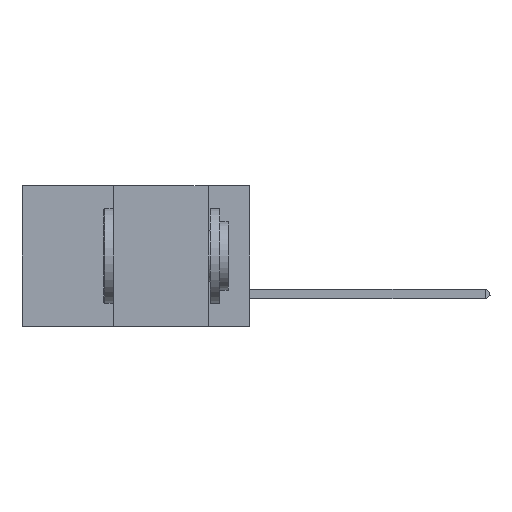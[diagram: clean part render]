
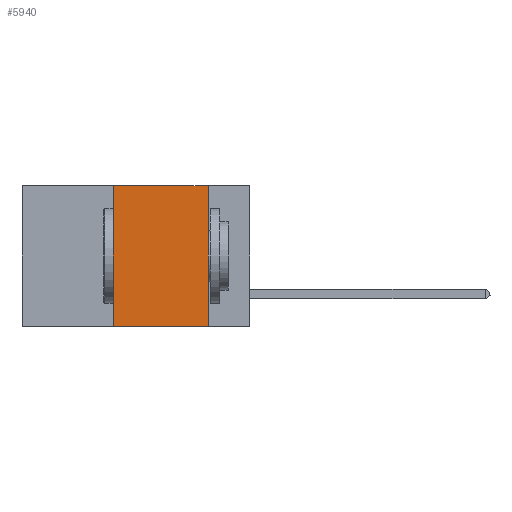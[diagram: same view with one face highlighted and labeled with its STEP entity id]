
A CAD part, left-side view. The second image highlights one B-rep face of the part: STEP entity #5940.
In plain terms, the highlighted planar face has unit normal (-1, 0, 0).
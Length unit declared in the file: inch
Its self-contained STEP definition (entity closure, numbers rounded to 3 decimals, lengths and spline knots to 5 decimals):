
#159 = DIRECTION ( 'NONE',  ( 0., -1., 0. ) ) ;
#1230 = CARTESIAN_POINT ( 'NONE',  ( 0., 0.6, -0.37 ) ) ;
#1300 = VERTEX_POINT ( 'NONE', #4071 ) ;
#1934 = DIRECTION ( 'NONE',  ( 0., 0., -1. ) ) ;
#2097 = CARTESIAN_POINT ( 'NONE',  ( 0., 0.11, -0.37 ) ) ;
#2339 = VERTEX_POINT ( 'NONE', #17075 ) ;
#2477 = ORIENTED_EDGE ( 'NONE', *, *, #18379, .T. ) ;
#2671 = LINE ( 'NONE', #12199, #7396 ) ;
#2758 = DIRECTION ( 'NONE',  ( 0., 0., -1. ) ) ;
#2958 = DIRECTION ( 'NONE',  ( 0., 0., 1. ) ) ;
#3792 = DIRECTION ( 'NONE',  ( 1., 0., 0. ) ) ;
#4071 = CARTESIAN_POINT ( 'NONE',  ( 0., 0.11, 0. ) ) ;
#4205 = VERTEX_POINT ( 'NONE', #18682 ) ;
#4425 = DIRECTION ( 'NONE',  ( 0., -1., 0. ) ) ;
#5059 = ORIENTED_EDGE ( 'NONE', *, *, #13783, .F. ) ;
#5210 = CARTESIAN_POINT ( 'NONE',  ( 0., 0.11, 0. ) ) ;
#5594 = FACE_OUTER_BOUND ( 'NONE', #8528, .T. ) ;
#5718 = LINE ( 'NONE', #5210, #13878 ) ;
#5916 = VERTEX_POINT ( 'NONE', #2097 ) ;
#5940 = ADVANCED_FACE ( 'NONE', ( #5594 ), #11528, .F. ) ;
#6797 = LINE ( 'NONE', #9193, #7574 ) ;
#7396 = VECTOR ( 'NONE', #159, 39.37008 ) ;
#7574 = VECTOR ( 'NONE', #2958, 39.37008 ) ;
#8528 = EDGE_LOOP ( 'NONE', ( #9551, #5059, #19183, #2477 ) ) ;
#9193 = CARTESIAN_POINT ( 'NONE',  ( 0., 0.36, 0. ) ) ;
#9296 = LINE ( 'NONE', #1230, #12015 ) ;
#9551 = ORIENTED_EDGE ( 'NONE', *, *, #17405, .F. ) ;
#11528 = PLANE ( 'NONE',  #12906 ) ;
#12015 = VECTOR ( 'NONE', #4425, 39.37008 ) ;
#12199 = CARTESIAN_POINT ( 'NONE',  ( 0., 0.6, 0. ) ) ;
#12906 = AXIS2_PLACEMENT_3D ( 'NONE', #13106, #3792, #2758 ) ;
#13106 = CARTESIAN_POINT ( 'NONE',  ( 0., 0.6, 0. ) ) ;
#13783 = EDGE_CURVE ( 'NONE', #2339, #1300, #2671, .T. ) ;
#13878 = VECTOR ( 'NONE', #1934, 39.37008 ) ;
#17075 = CARTESIAN_POINT ( 'NONE',  ( 0., 0.36, 0. ) ) ;
#17405 = EDGE_CURVE ( 'NONE', #1300, #5916, #5718, .T. ) ;
#18379 = EDGE_CURVE ( 'NONE', #4205, #5916, #9296, .T. ) ;
#18628 = EDGE_CURVE ( 'NONE', #4205, #2339, #6797, .T. ) ;
#18682 = CARTESIAN_POINT ( 'NONE',  ( 0., 0.36, -0.37 ) ) ;
#19183 = ORIENTED_EDGE ( 'NONE', *, *, #18628, .F. ) ;
